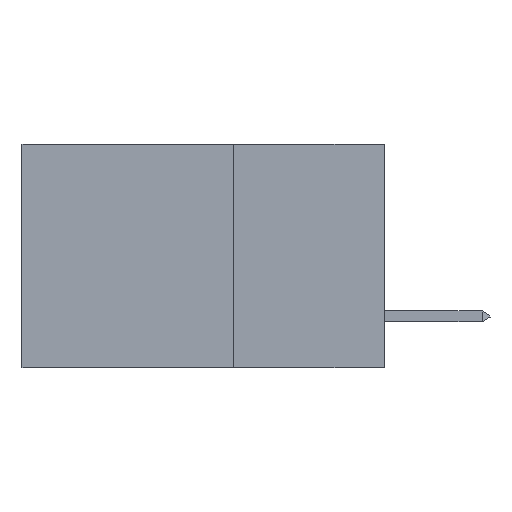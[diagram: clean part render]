
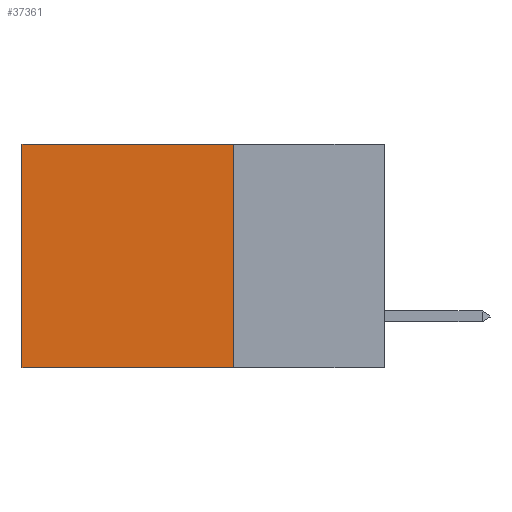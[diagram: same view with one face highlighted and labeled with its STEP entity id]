
A CAD part, left-side view. The second image highlights one B-rep face of the part: STEP entity #37361.
In plain terms, the highlighted planar face has unit normal (-1, 0, 0).
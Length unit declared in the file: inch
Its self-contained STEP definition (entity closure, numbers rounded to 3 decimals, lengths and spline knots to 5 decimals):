
#177 = LINE ( 'NONE', #4478, #36454 ) ;
#858 = VERTEX_POINT ( 'NONE', #42421 ) ;
#973 = EDGE_LOOP ( 'NONE', ( #29825, #15631, #36050, #22617 ) ) ;
#4478 = CARTESIAN_POINT ( 'NONE',  ( 0.2875, 0.25, 0. ) ) ;
#7153 = VECTOR ( 'NONE', #35830, 39.37008 ) ;
#7467 = PLANE ( 'NONE',  #34163 ) ;
#8736 = VECTOR ( 'NONE', #20016, 39.37008 ) ;
#10224 = CARTESIAN_POINT ( 'NONE',  ( 0.2875, 0.6, -0.37 ) ) ;
#10303 = CARTESIAN_POINT ( 'NONE',  ( 0.2875, 0.25, -0.37 ) ) ;
#11417 = DIRECTION ( 'NONE',  ( 1., 0., 0. ) ) ;
#12729 = VERTEX_POINT ( 'NONE', #37429 ) ;
#15114 = LINE ( 'NONE', #35536, #43812 ) ;
#15631 = ORIENTED_EDGE ( 'NONE', *, *, #27635, .F. ) ;
#16285 = FACE_OUTER_BOUND ( 'NONE', #973, .T. ) ;
#18524 = LINE ( 'NONE', #10303, #7153 ) ;
#19342 = VERTEX_POINT ( 'NONE', #21640 ) ;
#20016 = DIRECTION ( 'NONE',  ( 0., 0., -1. ) ) ;
#21640 = CARTESIAN_POINT ( 'NONE',  ( 0.2875, 0.25, 0. ) ) ;
#22617 = ORIENTED_EDGE ( 'NONE', *, *, #39413, .T. ) ;
#25233 = DIRECTION ( 'NONE',  ( 0., 0., -1. ) ) ;
#25742 = DIRECTION ( 'NONE',  ( 0., 1., 0. ) ) ;
#27635 = EDGE_CURVE ( 'NONE', #12729, #42853, #18524, .T. ) ;
#28626 = CARTESIAN_POINT ( 'NONE',  ( 0.2875, 0.25, 0. ) ) ;
#29825 = ORIENTED_EDGE ( 'NONE', *, *, #37473, .T. ) ;
#30928 = LINE ( 'NONE', #40714, #8736 ) ;
#34163 = AXIS2_PLACEMENT_3D ( 'NONE', #28626, #11417, #35606 ) ;
#35536 = CARTESIAN_POINT ( 'NONE',  ( 0.2875, 0.25, 0. ) ) ;
#35606 = DIRECTION ( 'NONE',  ( 0., 0., -1. ) ) ;
#35830 = DIRECTION ( 'NONE',  ( 0., 1., 0. ) ) ;
#36050 = ORIENTED_EDGE ( 'NONE', *, *, #43895, .F. ) ;
#36454 = VECTOR ( 'NONE', #25233, 39.37008 ) ;
#37361 = ADVANCED_FACE ( 'NONE', ( #16285 ), #7467, .F. ) ;
#37429 = CARTESIAN_POINT ( 'NONE',  ( 0.2875, 0.25, -0.37 ) ) ;
#37473 = EDGE_CURVE ( 'NONE', #858, #42853, #30928, .T. ) ;
#39413 = EDGE_CURVE ( 'NONE', #19342, #858, #15114, .T. ) ;
#40714 = CARTESIAN_POINT ( 'NONE',  ( 0.2875, 0.6, 0. ) ) ;
#42421 = CARTESIAN_POINT ( 'NONE',  ( 0.2875, 0.6, 0. ) ) ;
#42853 = VERTEX_POINT ( 'NONE', #10224 ) ;
#43812 = VECTOR ( 'NONE', #25742, 39.37008 ) ;
#43895 = EDGE_CURVE ( 'NONE', #19342, #12729, #177, .T. ) ;
